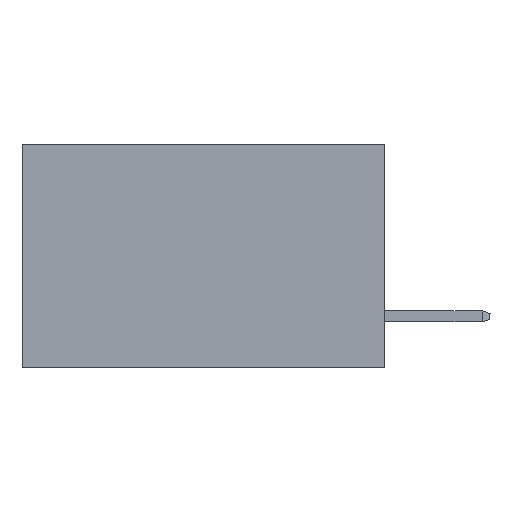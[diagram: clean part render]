
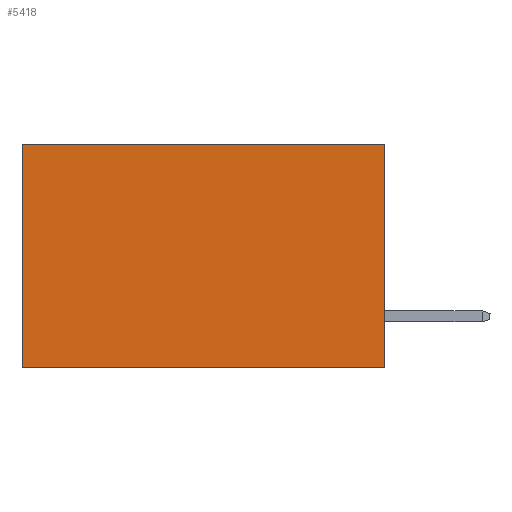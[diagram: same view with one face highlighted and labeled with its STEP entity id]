
A CAD part, left-side view. The second image highlights one B-rep face of the part: STEP entity #5418.
In plain terms, the highlighted planar face has unit normal (-1, 0, 0).
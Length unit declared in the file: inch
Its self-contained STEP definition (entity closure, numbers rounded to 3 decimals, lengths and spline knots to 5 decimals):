
#370 = VECTOR ( 'NONE', #10893, 39.37008 ) ;
#489 = LINE ( 'NONE', #10644, #8397 ) ;
#1281 = VECTOR ( 'NONE', #6521, 39.37008 ) ;
#1475 = LINE ( 'NONE', #2351, #370 ) ;
#1545 = CARTESIAN_POINT ( 'NONE',  ( 0.2615, 0., 0. ) ) ;
#1571 = CARTESIAN_POINT ( 'NONE',  ( 0.2615, 0.6, 0. ) ) ;
#2074 = DIRECTION ( 'NONE',  ( 0., 1., 0. ) ) ;
#2178 = AXIS2_PLACEMENT_3D ( 'NONE', #2429, #7819, #5261 ) ;
#2351 = CARTESIAN_POINT ( 'NONE',  ( 0.2615, 0., -0.37 ) ) ;
#2429 = CARTESIAN_POINT ( 'NONE',  ( 0.2615, 0., -0.37 ) ) ;
#2923 = EDGE_CURVE ( 'NONE', #9776, #4476, #7535, .T. ) ;
#3218 = VECTOR ( 'NONE', #2074, 39.37008 ) ;
#3518 = ORIENTED_EDGE ( 'NONE', *, *, #10018, .F. ) ;
#3665 = DIRECTION ( 'NONE',  ( 0., 0., -1. ) ) ;
#3780 = ORIENTED_EDGE ( 'NONE', *, *, #2923, .F. ) ;
#4062 = CARTESIAN_POINT ( 'NONE',  ( 0.2615, 0., -0.37 ) ) ;
#4476 = VERTEX_POINT ( 'NONE', #4062 ) ;
#5261 = DIRECTION ( 'NONE',  ( 0., 0., -1. ) ) ;
#5418 = ADVANCED_FACE ( 'NONE', ( #6665 ), #10072, .F. ) ;
#5525 = CARTESIAN_POINT ( 'NONE',  ( 0.2615, 0.6, -0.37 ) ) ;
#6325 = VERTEX_POINT ( 'NONE', #1571 ) ;
#6521 = DIRECTION ( 'NONE',  ( 0., 0., -1. ) ) ;
#6665 = FACE_OUTER_BOUND ( 'NONE', #8006, .T. ) ;
#7142 = CARTESIAN_POINT ( 'NONE',  ( 0.2615, 0., 0. ) ) ;
#7397 = ORIENTED_EDGE ( 'NONE', *, *, #8257, .T. ) ;
#7535 = LINE ( 'NONE', #10139, #1281 ) ;
#7819 = DIRECTION ( 'NONE',  ( 1., 0., 0. ) ) ;
#8006 = EDGE_LOOP ( 'NONE', ( #7397, #3518, #3780, #9528 ) ) ;
#8257 = EDGE_CURVE ( 'NONE', #6325, #8639, #489, .T. ) ;
#8397 = VECTOR ( 'NONE', #3665, 39.37008 ) ;
#8621 = EDGE_CURVE ( 'NONE', #9776, #6325, #8890, .T. ) ;
#8639 = VERTEX_POINT ( 'NONE', #5525 ) ;
#8890 = LINE ( 'NONE', #7142, #3218 ) ;
#9528 = ORIENTED_EDGE ( 'NONE', *, *, #8621, .T. ) ;
#9776 = VERTEX_POINT ( 'NONE', #1545 ) ;
#10018 = EDGE_CURVE ( 'NONE', #4476, #8639, #1475, .T. ) ;
#10072 = PLANE ( 'NONE',  #2178 ) ;
#10139 = CARTESIAN_POINT ( 'NONE',  ( 0.2615, 0., -0.37 ) ) ;
#10644 = CARTESIAN_POINT ( 'NONE',  ( 0.2615, 0.6, -0.37 ) ) ;
#10893 = DIRECTION ( 'NONE',  ( 0., 1., 0. ) ) ;
